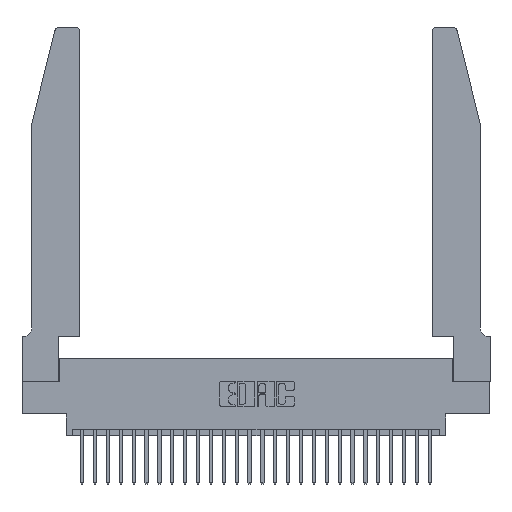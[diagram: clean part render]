
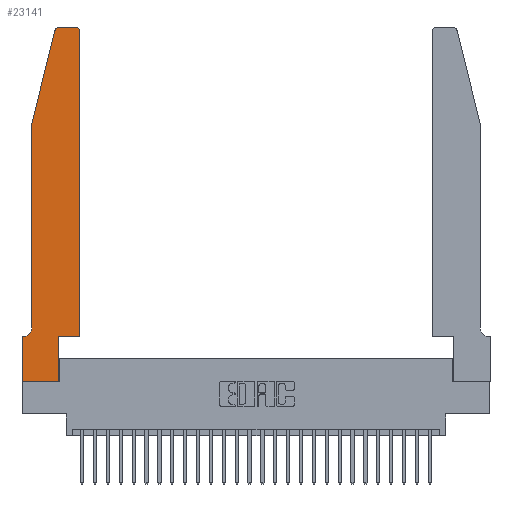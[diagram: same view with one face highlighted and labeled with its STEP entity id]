
A CAD part, top view. The second image highlights one B-rep face of the part: STEP entity #23141.
In plain terms, the highlighted planar face has unit normal (0, 0, 1).
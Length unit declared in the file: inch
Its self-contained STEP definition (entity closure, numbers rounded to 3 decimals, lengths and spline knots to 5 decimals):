
#57 = DIRECTION ( 'NONE',  ( 0., -1., 0. ) ) ;
#116 = VECTOR ( 'NONE', #18788, 39.37008 ) ;
#457 = ORIENTED_EDGE ( 'NONE', *, *, #18897, .T. ) ;
#556 = VECTOR ( 'NONE', #57, 39.37008 ) ;
#593 = DIRECTION ( 'NONE',  ( 1., 0., 0. ) ) ;
#598 = CARTESIAN_POINT ( 'NONE',  ( 0.4205, 2.72, 0.37 ) ) ;
#1015 = ORIENTED_EDGE ( 'NONE', *, *, #2451, .T. ) ;
#1783 = CARTESIAN_POINT ( 'NONE',  ( 0.4505, 0.35, 0.37 ) ) ;
#2451 = EDGE_CURVE ( 'NONE', #15192, #6120, #17483, .T. ) ;
#2802 = DIRECTION ( 'NONE',  ( 0., 0., 1. ) ) ;
#2901 = CARTESIAN_POINT ( 'NONE',  ( 0.2865, 0.35, 0.37 ) ) ;
#2942 = ORIENTED_EDGE ( 'NONE', *, *, #10738, .T. ) ;
#2949 = DIRECTION ( 'NONE',  ( 1., 0., 0. ) ) ;
#3371 = EDGE_CURVE ( 'NONE', #13198, #7035, #18759, .T. ) ;
#3738 = LINE ( 'NONE', #18624, #9830 ) ;
#4045 = VERTEX_POINT ( 'NONE', #23938 ) ;
#4470 = CARTESIAN_POINT ( 'NONE',  ( 0., 0.35, 0.37 ) ) ;
#5318 = EDGE_CURVE ( 'NONE', #5986, #15192, #24425, .T. ) ;
#5556 = FACE_OUTER_BOUND ( 'NONE', #17873, .T. ) ;
#5653 = VECTOR ( 'NONE', #16208, 39.37008 ) ;
#5977 = VERTEX_POINT ( 'NONE', #12044 ) ;
#5986 = VERTEX_POINT ( 'NONE', #27373 ) ;
#6120 = VERTEX_POINT ( 'NONE', #12718 ) ;
#6488 = CARTESIAN_POINT ( 'NONE',  ( 0.0055, 0.42, 0.37 ) ) ;
#6779 = DIRECTION ( 'NONE',  ( 1., 0., 0. ) ) ;
#7035 = VERTEX_POINT ( 'NONE', #24666 ) ;
#7078 = ORIENTED_EDGE ( 'NONE', *, *, #8997, .T. ) ;
#7281 = AXIS2_PLACEMENT_3D ( 'NONE', #598, #16462, #2949 ) ;
#8795 = DIRECTION ( 'NONE',  ( -1., 0., 0. ) ) ;
#8997 = EDGE_CURVE ( 'NONE', #13744, #23518, #3738, .T. ) ;
#9082 = AXIS2_PLACEMENT_3D ( 'NONE', #16336, #2802, #18489 ) ;
#9316 = CARTESIAN_POINT ( 'NONE',  ( 0., 0., 0.37 ) ) ;
#9830 = VECTOR ( 'NONE', #593, 39.37008 ) ;
#9899 = VECTOR ( 'NONE', #22868, 39.37008 ) ;
#10072 = ORIENTED_EDGE ( 'NONE', *, *, #3371, .T. ) ;
#10738 = EDGE_CURVE ( 'NONE', #4045, #17371, #13225, .T. ) ;
#10764 = CIRCLE ( 'NONE', #13028, 0.07 ) ;
#11077 = LINE ( 'NONE', #26742, #22706 ) ;
#11307 = LINE ( 'NONE', #25825, #17163 ) ;
#11992 = DIRECTION ( 'NONE',  ( -1., 0., 0. ) ) ;
#12020 = LINE ( 'NONE', #13824, #556 ) ;
#12044 = CARTESIAN_POINT ( 'NONE',  ( 0.0055, 0.35, 0.37 ) ) ;
#12275 = CARTESIAN_POINT ( 'NONE',  ( 0.0755, 2., 0.37 ) ) ;
#12373 = ORIENTED_EDGE ( 'NONE', *, *, #28340, .T. ) ;
#12380 = LINE ( 'NONE', #24831, #5653 ) ;
#12600 = ORIENTED_EDGE ( 'NONE', *, *, #28105, .T. ) ;
#12718 = CARTESIAN_POINT ( 'NONE',  ( 0.0755, 2., 0.37 ) ) ;
#12947 = VECTOR ( 'NONE', #26243, 39.37008 ) ;
#13028 = AXIS2_PLACEMENT_3D ( 'NONE', #6488, #21994, #8795 ) ;
#13132 = ORIENTED_EDGE ( 'NONE', *, *, #22073, .T. ) ;
#13198 = VERTEX_POINT ( 'NONE', #20635 ) ;
#13225 = CIRCLE ( 'NONE', #7281, 0.03 ) ;
#13744 = VERTEX_POINT ( 'NONE', #9316 ) ;
#13824 = CARTESIAN_POINT ( 'NONE',  ( 0., 0., 0.37 ) ) ;
#13942 = ORIENTED_EDGE ( 'NONE', *, *, #16879, .T. ) ;
#14089 = AXIS2_PLACEMENT_3D ( 'NONE', #4470, #20096, #6779 ) ;
#15192 = VERTEX_POINT ( 'NONE', #18673 ) ;
#15518 = EDGE_CURVE ( 'NONE', #23625, #5977, #10764, .T. ) ;
#15708 = PLANE ( 'NONE',  #14089 ) ;
#16208 = DIRECTION ( 'NONE',  ( 0., -1., 0. ) ) ;
#16327 = CARTESIAN_POINT ( 'NONE',  ( 0.4205, 2.75, 0.37 ) ) ;
#16336 = CARTESIAN_POINT ( 'NONE',  ( 0.284, 2.72, 0.37 ) ) ;
#16443 = CARTESIAN_POINT ( 'NONE',  ( 0.0755, 0.35, 0.37 ) ) ;
#16462 = DIRECTION ( 'NONE',  ( 0., 0., 1. ) ) ;
#16575 = VERTEX_POINT ( 'NONE', #21387 ) ;
#16879 = EDGE_CURVE ( 'NONE', #7035, #4045, #11077, .T. ) ;
#17163 = VECTOR ( 'NONE', #27880, 39.37008 ) ;
#17371 = VERTEX_POINT ( 'NONE', #16327 ) ;
#17483 = LINE ( 'NONE', #12275, #116 ) ;
#17547 = ORIENTED_EDGE ( 'NONE', *, *, #5318, .T. ) ;
#17873 = EDGE_LOOP ( 'NONE', ( #457, #17547, #1015, #12600, #19060, #18423, #12373, #7078, #13132, #10072, #13942, #2942 ) ) ;
#18423 = ORIENTED_EDGE ( 'NONE', *, *, #24060, .T. ) ;
#18489 = DIRECTION ( 'NONE',  ( 1., 0., 0. ) ) ;
#18624 = CARTESIAN_POINT ( 'NONE',  ( 0., 0., 0.37 ) ) ;
#18673 = CARTESIAN_POINT ( 'NONE',  ( 0.25487, 2.72718, 0.37 ) ) ;
#18759 = LINE ( 'NONE', #1783, #12947 ) ;
#18788 = DIRECTION ( 'NONE',  ( -0.239, -0.971, 0. ) ) ;
#18897 = EDGE_CURVE ( 'NONE', #17371, #5986, #11307, .T. ) ;
#19060 = ORIENTED_EDGE ( 'NONE', *, *, #15518, .T. ) ;
#20096 = DIRECTION ( 'NONE',  ( 0., 0., 1. ) ) ;
#20322 = DIRECTION ( 'NONE',  ( 0., 1., 0. ) ) ;
#20635 = CARTESIAN_POINT ( 'NONE',  ( 0.2865, 0.35, 0.37 ) ) ;
#20926 = LINE ( 'NONE', #2901, #9899 ) ;
#21387 = CARTESIAN_POINT ( 'NONE',  ( 0., 0.35, 0.37 ) ) ;
#21597 = CARTESIAN_POINT ( 'NONE',  ( 0.0755, 0.42, 0.37 ) ) ;
#21994 = DIRECTION ( 'NONE',  ( 0., 0., -1. ) ) ;
#22073 = EDGE_CURVE ( 'NONE', #23518, #13198, #20926, .T. ) ;
#22706 = VECTOR ( 'NONE', #20322, 39.37008 ) ;
#22868 = DIRECTION ( 'NONE',  ( 0., 1., 0. ) ) ;
#23141 = ADVANCED_FACE ( 'NONE', ( #5556 ), #15708, .T. ) ;
#23518 = VERTEX_POINT ( 'NONE', #25570 ) ;
#23625 = VERTEX_POINT ( 'NONE', #21597 ) ;
#23851 = LINE ( 'NONE', #16443, #27552 ) ;
#23938 = CARTESIAN_POINT ( 'NONE',  ( 0.4505, 2.72, 0.37 ) ) ;
#24060 = EDGE_CURVE ( 'NONE', #5977, #16575, #23851, .T. ) ;
#24425 = CIRCLE ( 'NONE', #9082, 0.03 ) ;
#24666 = CARTESIAN_POINT ( 'NONE',  ( 0.4505, 0.35, 0.37 ) ) ;
#24831 = CARTESIAN_POINT ( 'NONE',  ( 0.0755, 2., 0.37 ) ) ;
#25570 = CARTESIAN_POINT ( 'NONE',  ( 0.2865, 0., 0.37 ) ) ;
#25825 = CARTESIAN_POINT ( 'NONE',  ( 0.2605, 2.75, 0.37 ) ) ;
#26243 = DIRECTION ( 'NONE',  ( 1., 0., 0. ) ) ;
#26742 = CARTESIAN_POINT ( 'NONE',  ( 0.4505, 0.35, 0.37 ) ) ;
#27373 = CARTESIAN_POINT ( 'NONE',  ( 0.284, 2.75, 0.37 ) ) ;
#27552 = VECTOR ( 'NONE', #11992, 39.37008 ) ;
#27880 = DIRECTION ( 'NONE',  ( -1., 0., 0. ) ) ;
#28105 = EDGE_CURVE ( 'NONE', #6120, #23625, #12380, .T. ) ;
#28340 = EDGE_CURVE ( 'NONE', #16575, #13744, #12020, .T. ) ;
